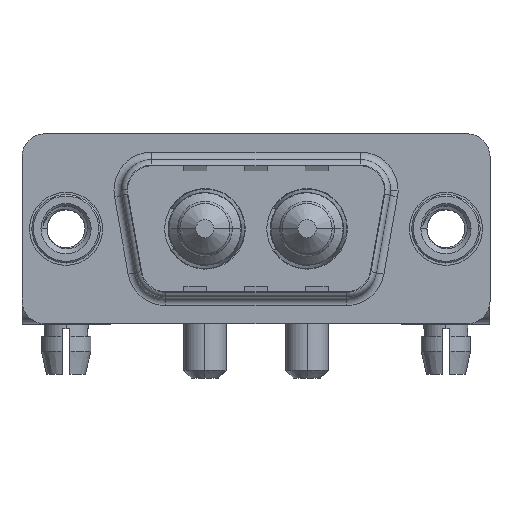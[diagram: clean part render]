
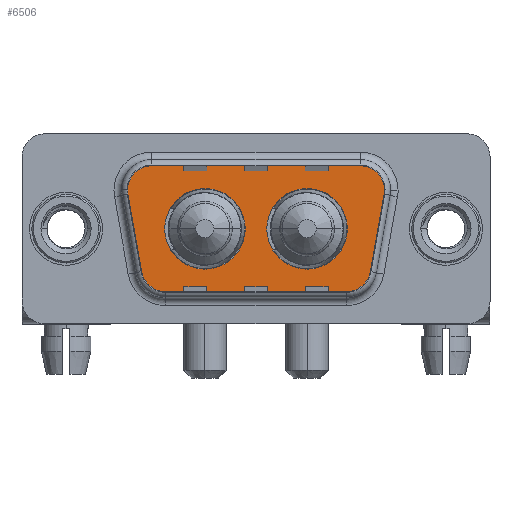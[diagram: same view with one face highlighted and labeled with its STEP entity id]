
A CAD part, top view. The second image highlights one B-rep face of the part: STEP entity #6506.
In plain terms, the highlighted planar face has unit normal (0, 0, 1).
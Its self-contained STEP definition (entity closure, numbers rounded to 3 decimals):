
#55 = LINE ( 'NONE', #13454, #4707 ) ;
#314 = EDGE_LOOP ( 'NONE', ( #7759, #10324, #11583, #13319, #2991, #4247, #375, #11527, #5057 ) ) ;
#375 = ORIENTED_EDGE ( 'NONE', *, *, #8096, .T. ) ;
#393 = DIRECTION ( 'NONE',  ( 0., 0., 1. ) ) ;
#616 = DIRECTION ( 'NONE',  ( -1., 0., 0. ) ) ;
#856 = VERTEX_POINT ( 'NONE', #12350 ) ;
#917 = DIRECTION ( 'NONE',  ( -1., 0., 0. ) ) ;
#1304 = CARTESIAN_POINT ( 'NONE',  ( 6.459, -4.9, 0. ) ) ;
#1459 = CARTESIAN_POINT ( 'NONE',  ( 6.49, 0., 0. ) ) ;
#1528 = AXIS2_PLACEMENT_3D ( 'NONE', #11694, #7885, #10503 ) ;
#1532 = EDGE_CURVE ( 'NONE', #6089, #10210, #11737, .T. ) ;
#1553 = DIRECTION ( 'NONE',  ( 0., 0., 1. ) ) ;
#1554 = CIRCLE ( 'NONE', #14988, 2.65 ) ;
#1564 = EDGE_CURVE ( 'NONE', #10210, #2395, #12218, .T. ) ;
#1710 = CARTESIAN_POINT ( 'NONE',  ( 19.564, 2.9, 0. ) ) ;
#2395 = VERTEX_POINT ( 'NONE', #9234 ) ;
#2563 = AXIS2_PLACEMENT_3D ( 'NONE', #6249, #11336, #11087 ) ;
#2689 = CIRCLE ( 'NONE', #10287, 2. ) ;
#2991 = ORIENTED_EDGE ( 'NONE', *, *, #5786, .T. ) ;
#3108 = EDGE_CURVE ( 'NONE', #4046, #8502, #5640, .T. ) ;
#3257 = VERTEX_POINT ( 'NONE', #14990 ) ;
#3275 = DIRECTION ( 'NONE',  ( 1., 0., 0. ) ) ;
#3374 = DIRECTION ( 'NONE',  ( 0., 0., 1. ) ) ;
#3416 = ORIENTED_EDGE ( 'NONE', *, *, #5092, .F. ) ;
#3553 = VECTOR ( 'NONE', #13537, 1000. ) ;
#3723 = CARTESIAN_POINT ( 'NONE',  ( 9.14, 0., 0. ) ) ;
#3829 = AXIS2_PLACEMENT_3D ( 'NONE', #11481, #6636, #616 ) ;
#3962 = CARTESIAN_POINT ( 'NONE',  ( 9.14, 0., 0. ) ) ;
#4046 = VERTEX_POINT ( 'NONE', #1459 ) ;
#4103 = LINE ( 'NONE', #12513, #3553 ) ;
#4247 = ORIENTED_EDGE ( 'NONE', *, *, #8839, .T. ) ;
#4248 = EDGE_CURVE ( 'NONE', #3257, #9108, #11149, .T. ) ;
#4405 = DIRECTION ( 'NONE',  ( 1., 0., 0. ) ) ;
#4513 = ORIENTED_EDGE ( 'NONE', *, *, #3108, .F. ) ;
#4707 = VECTOR ( 'NONE', #6155, 1000. ) ;
#4828 = VECTOR ( 'NONE', #14297, 1000. ) ;
#5057 = ORIENTED_EDGE ( 'NONE', *, *, #6982, .T. ) ;
#5092 = EDGE_CURVE ( 'NONE', #8502, #4046, #9573, .T. ) ;
#5151 = FACE_OUTER_BOUND ( 'NONE', #314, .T. ) ;
#5640 = CIRCLE ( 'NONE', #11958, 2.65 ) ;
#5655 = CARTESIAN_POINT ( 'NONE',  ( 21.534, 2.553, 0. ) ) ;
#5786 = EDGE_CURVE ( 'NONE', #2395, #12447, #15435, .T. ) ;
#6089 = VERTEX_POINT ( 'NONE', #11275 ) ;
#6155 = DIRECTION ( 'NONE',  ( 0.174, -0.985, 0. ) ) ;
#6237 = VERTEX_POINT ( 'NONE', #12788 ) ;
#6249 = CARTESIAN_POINT ( 'NONE',  ( 18.541, -2.9, 0. ) ) ;
#6327 = FACE_BOUND ( 'NONE', #8151, .T. ) ;
#6494 = FACE_BOUND ( 'NONE', #7003, .T. ) ;
#6506 = ADVANCED_FACE ( 'NONE', ( #6327, #6494, #5151 ), #6571, .T. ) ;
#6571 = PLANE ( 'NONE',  #2563 ) ;
#6636 = DIRECTION ( 'NONE',  ( 0., 0., 1. ) ) ;
#6982 = EDGE_CURVE ( 'NONE', #15230, #3257, #4103, .T. ) ;
#7003 = EDGE_LOOP ( 'NONE', ( #3416, #4513 ) ) ;
#7017 = CARTESIAN_POINT ( 'NONE',  ( 21.564, 2.9, 0. ) ) ;
#7116 = EDGE_CURVE ( 'NONE', #6237, #15230, #12184, .T. ) ;
#7298 = AXIS2_PLACEMENT_3D ( 'NONE', #3962, #393, #12446 ) ;
#7341 = VERTEX_POINT ( 'NONE', #8153 ) ;
#7633 = EDGE_CURVE ( 'NONE', #9108, #6089, #9135, .T. ) ;
#7759 = ORIENTED_EDGE ( 'NONE', *, *, #4248, .T. ) ;
#7885 = DIRECTION ( 'NONE',  ( 0., 0., 1. ) ) ;
#8096 = EDGE_CURVE ( 'NONE', #856, #6237, #55, .T. ) ;
#8151 = EDGE_LOOP ( 'NONE', ( #13802, #9841 ) ) ;
#8153 = CARTESIAN_POINT ( 'NONE',  ( 13.21, 0., 0. ) ) ;
#8231 = CARTESIAN_POINT ( 'NONE',  ( 11.79, 0., 0. ) ) ;
#8381 = CARTESIAN_POINT ( 'NONE',  ( 18.51, 0., 0. ) ) ;
#8392 = AXIS2_PLACEMENT_3D ( 'NONE', #9229, #15104, #10410 ) ;
#8502 = VERTEX_POINT ( 'NONE', #8231 ) ;
#8839 = EDGE_CURVE ( 'NONE', #12447, #856, #2689, .T. ) ;
#9058 = CARTESIAN_POINT ( 'NONE',  ( 15.86, 0., 0. ) ) ;
#9108 = VERTEX_POINT ( 'NONE', #13574 ) ;
#9135 = LINE ( 'NONE', #5655, #4828 ) ;
#9229 = CARTESIAN_POINT ( 'NONE',  ( 15.86, 0., 0. ) ) ;
#9234 = CARTESIAN_POINT ( 'NONE',  ( 19.564, 4.9, 0. ) ) ;
#9327 = CARTESIAN_POINT ( 'NONE',  ( 5.436, 4.9, 0. ) ) ;
#9472 = CARTESIAN_POINT ( 'NONE',  ( 5.436, 2.9, 0. ) ) ;
#9573 = CIRCLE ( 'NONE', #7298, 2.65 ) ;
#9841 = ORIENTED_EDGE ( 'NONE', *, *, #14656, .F. ) ;
#9952 = DIRECTION ( 'NONE',  ( 0., 0., 1. ) ) ;
#10210 = VERTEX_POINT ( 'NONE', #7017 ) ;
#10212 = AXIS2_PLACEMENT_3D ( 'NONE', #13676, #9952, #14801 ) ;
#10287 = AXIS2_PLACEMENT_3D ( 'NONE', #9472, #3374, #4405 ) ;
#10324 = ORIENTED_EDGE ( 'NONE', *, *, #7633, .T. ) ;
#10410 = DIRECTION ( 'NONE',  ( 1., 0., 0. ) ) ;
#10503 = DIRECTION ( 'NONE',  ( 1., 0., 0. ) ) ;
#11087 = DIRECTION ( 'NONE',  ( 1., 0., 0. ) ) ;
#11149 = CIRCLE ( 'NONE', #1528, 2. ) ;
#11275 = CARTESIAN_POINT ( 'NONE',  ( 21.534, 2.553, 0. ) ) ;
#11336 = DIRECTION ( 'NONE',  ( 0., 0., 1. ) ) ;
#11467 = DIRECTION ( 'NONE',  ( -1., 0., 0. ) ) ;
#11481 = CARTESIAN_POINT ( 'NONE',  ( 6.459, -2.9, 0. ) ) ;
#11527 = ORIENTED_EDGE ( 'NONE', *, *, #7116, .T. ) ;
#11583 = ORIENTED_EDGE ( 'NONE', *, *, #1532, .T. ) ;
#11694 = CARTESIAN_POINT ( 'NONE',  ( 18.541, -2.9, 0. ) ) ;
#11699 = CARTESIAN_POINT ( 'NONE',  ( 5.436, 4.9, 0. ) ) ;
#11737 = CIRCLE ( 'NONE', #13481, 2. ) ;
#11844 = VERTEX_POINT ( 'NONE', #8381 ) ;
#11879 = VECTOR ( 'NONE', #917, 1000. ) ;
#11958 = AXIS2_PLACEMENT_3D ( 'NONE', #3723, #13236, #15638 ) ;
#12184 = CIRCLE ( 'NONE', #3829, 2. ) ;
#12192 = CIRCLE ( 'NONE', #8392, 2.65 ) ;
#12218 = CIRCLE ( 'NONE', #10212, 2. ) ;
#12350 = CARTESIAN_POINT ( 'NONE',  ( 3.466, 2.553, 0. ) ) ;
#12446 = DIRECTION ( 'NONE',  ( 1., 0., 0. ) ) ;
#12447 = VERTEX_POINT ( 'NONE', #9327 ) ;
#12513 = CARTESIAN_POINT ( 'NONE',  ( 6.459, -4.9, 0. ) ) ;
#12788 = CARTESIAN_POINT ( 'NONE',  ( 4.489, -3.247, 0. ) ) ;
#13236 = DIRECTION ( 'NONE',  ( 0., 0., 1. ) ) ;
#13319 = ORIENTED_EDGE ( 'NONE', *, *, #1564, .T. ) ;
#13454 = CARTESIAN_POINT ( 'NONE',  ( 3.466, 2.553, 0. ) ) ;
#13481 = AXIS2_PLACEMENT_3D ( 'NONE', #1710, #1553, #11467 ) ;
#13537 = DIRECTION ( 'NONE',  ( 1., 0., 0. ) ) ;
#13574 = CARTESIAN_POINT ( 'NONE',  ( 20.511, -3.247, 0. ) ) ;
#13676 = CARTESIAN_POINT ( 'NONE',  ( 19.564, 2.9, 0. ) ) ;
#13802 = ORIENTED_EDGE ( 'NONE', *, *, #14633, .F. ) ;
#14297 = DIRECTION ( 'NONE',  ( 0.174, 0.985, 0. ) ) ;
#14633 = EDGE_CURVE ( 'NONE', #11844, #7341, #12192, .T. ) ;
#14656 = EDGE_CURVE ( 'NONE', #7341, #11844, #1554, .T. ) ;
#14801 = DIRECTION ( 'NONE',  ( -1., 0., 0. ) ) ;
#14988 = AXIS2_PLACEMENT_3D ( 'NONE', #9058, #15180, #3275 ) ;
#14990 = CARTESIAN_POINT ( 'NONE',  ( 18.541, -4.9, 0. ) ) ;
#15104 = DIRECTION ( 'NONE',  ( 0., 0., 1. ) ) ;
#15180 = DIRECTION ( 'NONE',  ( 0., 0., 1. ) ) ;
#15230 = VERTEX_POINT ( 'NONE', #1304 ) ;
#15435 = LINE ( 'NONE', #11699, #11879 ) ;
#15638 = DIRECTION ( 'NONE',  ( 1., 0., 0. ) ) ;
